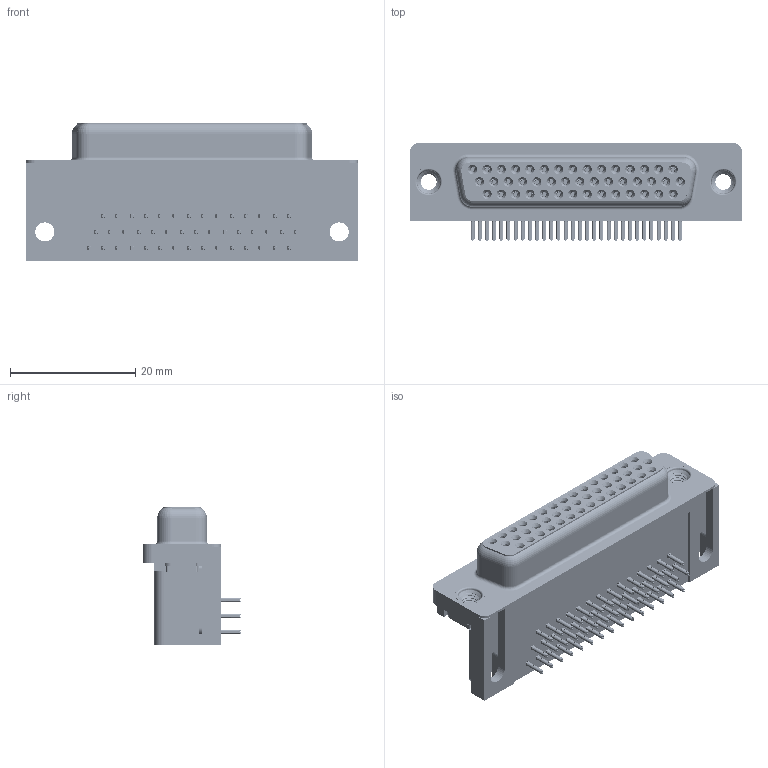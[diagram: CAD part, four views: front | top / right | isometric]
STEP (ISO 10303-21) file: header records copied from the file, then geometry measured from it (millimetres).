
FILE_DESCRIPTION (( 'STEP AP203' ), '1' );
FILE_NAME ('634-044-363-015.STEP', '2018-11-10T00:39:51', ( '' ), ( '' ), 'SwSTEP 2.0', 'SolidWorks 2016', '' );
FILE_SCHEMA (( 'CONFIG_CONTROL_DESIGN' ));
Length unit declared in the file: millimetre
Products named in the file (8): 634-044-363-015; 634 Housing_44 Socket; 634 Shell_44 Socket; Contact Bottom; Contact Middle; Contact Top; Thru Hole Board Mount; M3 Threaded Rivet
Assembly tree (50 placements, depth 2):
  634-044-363-015
    634 Housing_44 Socket
    634 Shell_44 Socket
    Contact Bottom  x14
    Contact Middle  x15
    Contact Top  x15
    Thru Hole Board Mount  x2
    M3 Threaded Rivet  x2
Bounding box: 53.04 x 15.73 x 22.1 mm (x, y, z)
Volume: 9349.4 mm3; surface area: 13270.6 mm2
Topology: 50 solids, 50 shells, 6535 faces, 17182 edges, 10784 vertices
Faces by surface type: plane 2927, bspline 1534, cylinder 1500, cone 536, torus 38
Entity records: 44395 total; most frequent: CARTESIAN_POINT 13218, ORIENTED_EDGE 6182, DIRECTION 5671, EDGE_CURVE 3091, LINE 2081, VECTOR 2081, VERTEX_POINT 1975, AXIS2_PLACEMENT_3D 1795
